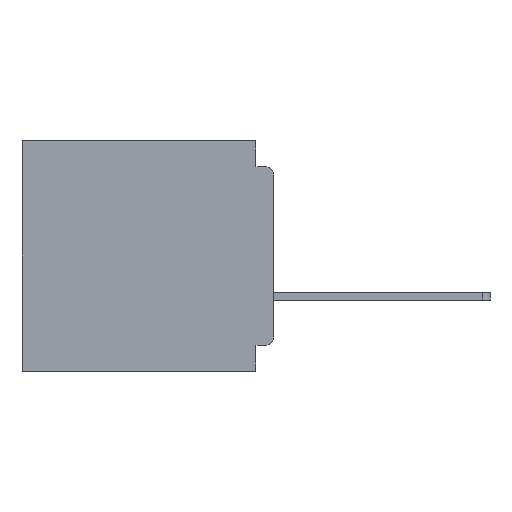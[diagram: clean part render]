
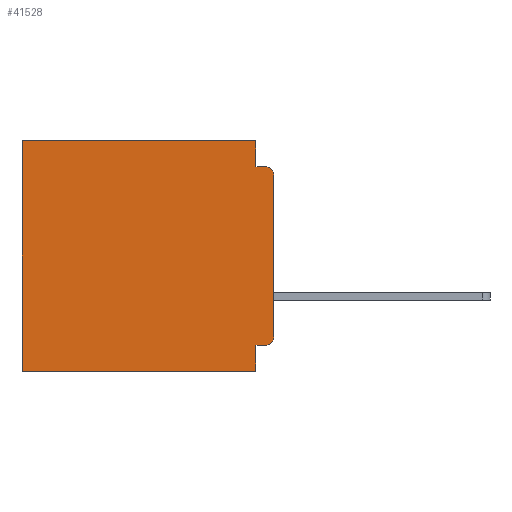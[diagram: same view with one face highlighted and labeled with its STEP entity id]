
A CAD part, left-side view. The second image highlights one B-rep face of the part: STEP entity #41528.
In plain terms, the highlighted planar face has unit normal (-1, 0, 0).
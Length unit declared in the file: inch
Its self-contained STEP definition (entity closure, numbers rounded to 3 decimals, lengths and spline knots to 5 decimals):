
#1720 = EDGE_LOOP ( 'NONE', ( #34648, #35884, #12083, #54392, #32374, #46665, #3414, #8433, #12947, #51035 ) ) ;
#2114 = VERTEX_POINT ( 'NONE', #16949 ) ;
#3033 = DIRECTION ( 'NONE',  ( 0., 0., -1. ) ) ;
#3414 = ORIENTED_EDGE ( 'NONE', *, *, #5647, .F. ) ;
#3817 = EDGE_CURVE ( 'NONE', #30196, #9871, #36174, .T. ) ;
#3957 = VERTEX_POINT ( 'NONE', #33279 ) ;
#4217 = AXIS2_PLACEMENT_3D ( 'NONE', #35750, #9542, #40116 ) ;
#4264 = EDGE_CURVE ( 'NONE', #23084, #2114, #46320, .T. ) ;
#5100 = CARTESIAN_POINT ( 'NONE',  ( 0.3, 0., -0.34 ) ) ;
#5647 = EDGE_CURVE ( 'NONE', #6303, #8346, #17534, .T. ) ;
#6303 = VERTEX_POINT ( 'NONE', #50864 ) ;
#7628 = LINE ( 'NONE', #55329, #52648 ) ;
#8182 = VECTOR ( 'NONE', #43176, 39.37008 ) ;
#8346 = VERTEX_POINT ( 'NONE', #54076 ) ;
#8433 = ORIENTED_EDGE ( 'NONE', *, *, #35718, .F. ) ;
#9542 = DIRECTION ( 'NONE',  ( -1., 0., 0. ) ) ;
#9739 = DIRECTION ( 'NONE',  ( 0., 0., -1. ) ) ;
#9871 = VERTEX_POINT ( 'NONE', #48056 ) ;
#10801 = CARTESIAN_POINT ( 'NONE',  ( 0.3, 0.015, -0.355 ) ) ;
#12083 = ORIENTED_EDGE ( 'NONE', *, *, #19359, .F. ) ;
#12619 = CARTESIAN_POINT ( 'NONE',  ( 0.3, 0.437, -0.4 ) ) ;
#12651 = CARTESIAN_POINT ( 'NONE',  ( 0.3, 0., -0.045 ) ) ;
#12947 = ORIENTED_EDGE ( 'NONE', *, *, #4264, .F. ) ;
#13519 = VECTOR ( 'NONE', #35300, 39.37008 ) ;
#16949 = CARTESIAN_POINT ( 'NONE',  ( 0.3, 0.031, -0.355 ) ) ;
#17534 = LINE ( 'NONE', #49484, #50896 ) ;
#19359 = EDGE_CURVE ( 'NONE', #3957, #9871, #43036, .T. ) ;
#19535 = EDGE_CURVE ( 'NONE', #23084, #44325, #32111, .T. ) ;
#19858 = EDGE_CURVE ( 'NONE', #46844, #3957, #27358, .T. ) ;
#20664 = CARTESIAN_POINT ( 'NONE',  ( 0.3, 0.031, 0. ) ) ;
#22792 = CARTESIAN_POINT ( 'NONE',  ( 0.3, 0., -0.355 ) ) ;
#22796 = CARTESIAN_POINT ( 'NONE',  ( 0.3, 0., -0.4 ) ) ;
#22968 = AXIS2_PLACEMENT_3D ( 'NONE', #38751, #36529, #39894 ) ;
#22985 = CARTESIAN_POINT ( 'NONE',  ( 0.3, 0., -0.4 ) ) ;
#23084 = VERTEX_POINT ( 'NONE', #10801 ) ;
#23188 = VECTOR ( 'NONE', #28834, 39.37008 ) ;
#23338 = VECTOR ( 'NONE', #56178, 39.37008 ) ;
#24224 = VECTOR ( 'NONE', #9739, 39.37008 ) ;
#25197 = LINE ( 'NONE', #44037, #13519 ) ;
#25580 = LINE ( 'NONE', #22985, #24224 ) ;
#25710 = CARTESIAN_POINT ( 'NONE',  ( 0.3, 0.437, 0. ) ) ;
#27208 = DIRECTION ( 'NONE',  ( 0., 0., -1. ) ) ;
#27358 = LINE ( 'NONE', #20664, #49090 ) ;
#28834 = DIRECTION ( 'NONE',  ( 0., 1., 0. ) ) ;
#30196 = VERTEX_POINT ( 'NONE', #47095 ) ;
#32111 = CIRCLE ( 'NONE', #4217, 0.015 ) ;
#32374 = ORIENTED_EDGE ( 'NONE', *, *, #50059, .T. ) ;
#33279 = CARTESIAN_POINT ( 'NONE',  ( 0.3, 0.031, -0.045 ) ) ;
#34648 = ORIENTED_EDGE ( 'NONE', *, *, #45577, .F. ) ;
#34909 = LINE ( 'NONE', #12619, #23338 ) ;
#35300 = DIRECTION ( 'NONE',  ( 0., 1., 0. ) ) ;
#35718 = EDGE_CURVE ( 'NONE', #2114, #6303, #7628, .T. ) ;
#35750 = CARTESIAN_POINT ( 'NONE',  ( 0.3, 0.015, -0.34 ) ) ;
#35884 = ORIENTED_EDGE ( 'NONE', *, *, #3817, .T. ) ;
#36174 = CIRCLE ( 'NONE', #22968, 0.015 ) ;
#36487 = EDGE_CURVE ( 'NONE', #39076, #8346, #34909, .T. ) ;
#36529 = DIRECTION ( 'NONE',  ( -1., 0., 0. ) ) ;
#38751 = CARTESIAN_POINT ( 'NONE',  ( 0.3, 0.015, -0.06 ) ) ;
#39076 = VERTEX_POINT ( 'NONE', #25710 ) ;
#39894 = DIRECTION ( 'NONE',  ( 0., 0., -1. ) ) ;
#40116 = DIRECTION ( 'NONE',  ( 0., 0., -1. ) ) ;
#40585 = FACE_OUTER_BOUND ( 'NONE', #1720, .T. ) ;
#40714 = CARTESIAN_POINT ( 'NONE',  ( 0.3, 0.031, 0. ) ) ;
#41528 = ADVANCED_FACE ( 'NONE', ( #40585 ), #44486, .F. ) ;
#43036 = LINE ( 'NONE', #12651, #8182 ) ;
#43176 = DIRECTION ( 'NONE',  ( 0., -1., 0. ) ) ;
#44037 = CARTESIAN_POINT ( 'NONE',  ( 0.3, 0., 0. ) ) ;
#44325 = VERTEX_POINT ( 'NONE', #5100 ) ;
#44486 = PLANE ( 'NONE',  #47441 ) ;
#45577 = EDGE_CURVE ( 'NONE', #30196, #44325, #25580, .T. ) ;
#46320 = LINE ( 'NONE', #22792, #23188 ) ;
#46665 = ORIENTED_EDGE ( 'NONE', *, *, #36487, .T. ) ;
#46844 = VERTEX_POINT ( 'NONE', #40714 ) ;
#47095 = CARTESIAN_POINT ( 'NONE',  ( 0.3, 0., -0.06 ) ) ;
#47441 = AXIS2_PLACEMENT_3D ( 'NONE', #22796, #53177, #27208 ) ;
#48056 = CARTESIAN_POINT ( 'NONE',  ( 0.3, 0.015, -0.045 ) ) ;
#49090 = VECTOR ( 'NONE', #3033, 39.37008 ) ;
#49484 = CARTESIAN_POINT ( 'NONE',  ( 0.3, 0., -0.4 ) ) ;
#50059 = EDGE_CURVE ( 'NONE', #46844, #39076, #25197, .T. ) ;
#50490 = DIRECTION ( 'NONE',  ( 0., 1., 0. ) ) ;
#50864 = CARTESIAN_POINT ( 'NONE',  ( 0.3, 0.031, -0.4 ) ) ;
#50896 = VECTOR ( 'NONE', #50490, 39.37008 ) ;
#51035 = ORIENTED_EDGE ( 'NONE', *, *, #19535, .T. ) ;
#51189 = DIRECTION ( 'NONE',  ( 0., 0., -1. ) ) ;
#52648 = VECTOR ( 'NONE', #51189, 39.37008 ) ;
#53177 = DIRECTION ( 'NONE',  ( 1., 0., 0. ) ) ;
#54076 = CARTESIAN_POINT ( 'NONE',  ( 0.3, 0.437, -0.4 ) ) ;
#54392 = ORIENTED_EDGE ( 'NONE', *, *, #19858, .F. ) ;
#55329 = CARTESIAN_POINT ( 'NONE',  ( 0.3, 0.031, -0.4 ) ) ;
#56178 = DIRECTION ( 'NONE',  ( 0., 0., -1. ) ) ;
